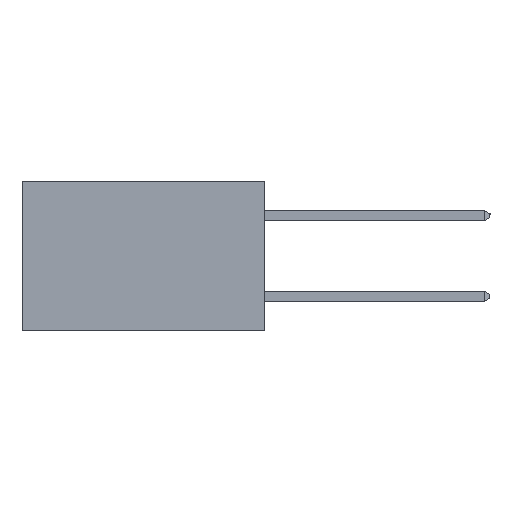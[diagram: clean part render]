
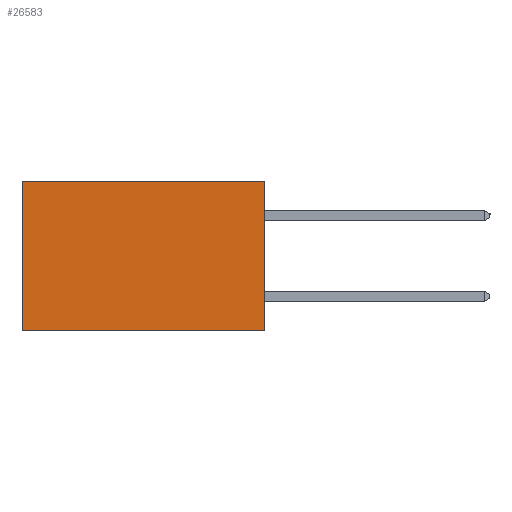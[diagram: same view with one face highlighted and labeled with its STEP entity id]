
A CAD part, left-side view. The second image highlights one B-rep face of the part: STEP entity #26583.
In plain terms, the highlighted planar face has unit normal (-1, 0, 0).
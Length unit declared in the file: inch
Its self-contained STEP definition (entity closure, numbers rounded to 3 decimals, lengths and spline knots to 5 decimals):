
#155 = EDGE_CURVE ( 'NONE', #19358, #13689, #25891, .T. ) ;
#1775 = AXIS2_PLACEMENT_3D ( 'NONE', #13868, #26597, #22437 ) ;
#2862 = VECTOR ( 'NONE', #15365, 39.37008 ) ;
#3920 = ORIENTED_EDGE ( 'NONE', *, *, #15541, .F. ) ;
#4604 = CARTESIAN_POINT ( 'NONE',  ( 0.2615, 0., 0. ) ) ;
#6332 = DIRECTION ( 'NONE',  ( 0., 1., 0. ) ) ;
#6954 = CARTESIAN_POINT ( 'NONE',  ( 0.2615, 0.6, -0.37 ) ) ;
#7527 = ORIENTED_EDGE ( 'NONE', *, *, #155, .T. ) ;
#7909 = CARTESIAN_POINT ( 'NONE',  ( 0.2615, 0.6, -0.37 ) ) ;
#8278 = DIRECTION ( 'NONE',  ( 0., 0., -1. ) ) ;
#8602 = LINE ( 'NONE', #21040, #13710 ) ;
#10395 = CARTESIAN_POINT ( 'NONE',  ( 0.2615, 0., -0.37 ) ) ;
#13443 = ORIENTED_EDGE ( 'NONE', *, *, #26748, .T. ) ;
#13689 = VERTEX_POINT ( 'NONE', #7909 ) ;
#13710 = VECTOR ( 'NONE', #25047, 39.37008 ) ;
#13868 = CARTESIAN_POINT ( 'NONE',  ( 0.2615, 0., -0.37 ) ) ;
#13986 = CARTESIAN_POINT ( 'NONE',  ( 0.2615, 0.6, 0. ) ) ;
#15365 = DIRECTION ( 'NONE',  ( 0., 0., -1. ) ) ;
#15541 = EDGE_CURVE ( 'NONE', #24390, #13689, #24867, .T. ) ;
#17816 = VERTEX_POINT ( 'NONE', #4604 ) ;
#19358 = VERTEX_POINT ( 'NONE', #13986 ) ;
#20007 = EDGE_CURVE ( 'NONE', #17816, #24390, #26823, .T. ) ;
#21040 = CARTESIAN_POINT ( 'NONE',  ( 0.2615, 0., 0. ) ) ;
#22437 = DIRECTION ( 'NONE',  ( 0., 0., -1. ) ) ;
#22693 = EDGE_LOOP ( 'NONE', ( #7527, #3920, #24707, #13443 ) ) ;
#23720 = VECTOR ( 'NONE', #8278, 39.37008 ) ;
#24390 = VERTEX_POINT ( 'NONE', #10395 ) ;
#24512 = FACE_OUTER_BOUND ( 'NONE', #22693, .T. ) ;
#24707 = ORIENTED_EDGE ( 'NONE', *, *, #20007, .F. ) ;
#24867 = LINE ( 'NONE', #25683, #26725 ) ;
#25047 = DIRECTION ( 'NONE',  ( 0., 1., 0. ) ) ;
#25683 = CARTESIAN_POINT ( 'NONE',  ( 0.2615, 0., -0.37 ) ) ;
#25891 = LINE ( 'NONE', #6954, #2862 ) ;
#26455 = PLANE ( 'NONE',  #1775 ) ;
#26583 = ADVANCED_FACE ( 'NONE', ( #24512 ), #26455, .F. ) ;
#26597 = DIRECTION ( 'NONE',  ( 1., 0., 0. ) ) ;
#26725 = VECTOR ( 'NONE', #6332, 39.37008 ) ;
#26748 = EDGE_CURVE ( 'NONE', #17816, #19358, #8602, .T. ) ;
#26823 = LINE ( 'NONE', #27228, #23720 ) ;
#27228 = CARTESIAN_POINT ( 'NONE',  ( 0.2615, 0., -0.37 ) ) ;
